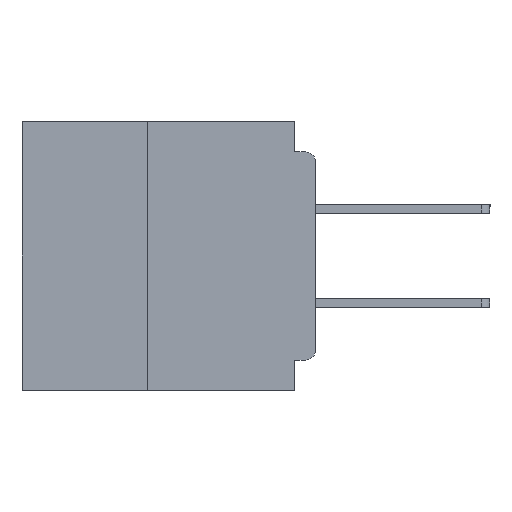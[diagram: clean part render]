
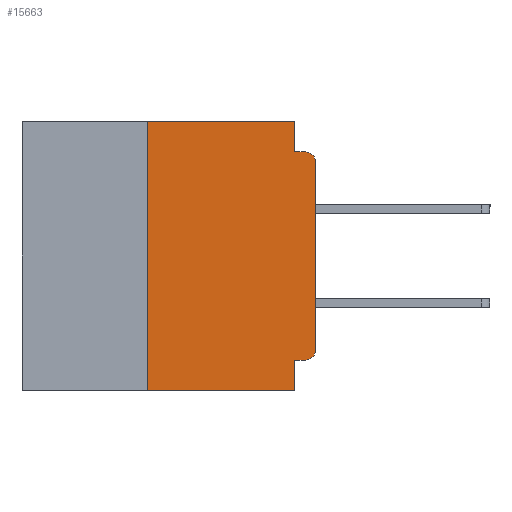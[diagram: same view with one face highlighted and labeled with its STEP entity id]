
A CAD part, left-side view. The second image highlights one B-rep face of the part: STEP entity #15663.
In plain terms, the highlighted planar face has unit normal (-1, 0, 0).
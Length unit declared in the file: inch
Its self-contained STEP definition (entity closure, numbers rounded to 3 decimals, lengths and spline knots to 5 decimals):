
#1507 = FACE_OUTER_BOUND ( 'NONE', #39905, .T. ) ;
#1745 = DIRECTION ( 'NONE',  ( 1., 0., 0. ) ) ;
#2138 = VERTEX_POINT ( 'NONE', #24121 ) ;
#3805 = CIRCLE ( 'NONE', #18743, 0.015 ) ;
#4704 = AXIS2_PLACEMENT_3D ( 'NONE', #35465, #9381, #39820 ) ;
#5245 = VECTOR ( 'NONE', #8273, 39.37008 ) ;
#5449 = VECTOR ( 'NONE', #32065, 39.37008 ) ;
#7479 = LINE ( 'NONE', #47610, #44870 ) ;
#7923 = CARTESIAN_POINT ( 'NONE',  ( 0., 0.031, -0.355 ) ) ;
#8273 = DIRECTION ( 'NONE',  ( 0., -1., 0. ) ) ;
#9055 = VERTEX_POINT ( 'NONE', #28958 ) ;
#9381 = DIRECTION ( 'NONE',  ( -1., 0., 0. ) ) ;
#9544 = VERTEX_POINT ( 'NONE', #45201 ) ;
#9561 = LINE ( 'NONE', #10356, #5449 ) ;
#9749 = ORIENTED_EDGE ( 'NONE', *, *, #20765, .T. ) ;
#10356 = CARTESIAN_POINT ( 'NONE',  ( 0., 0., -0.045 ) ) ;
#10501 = VECTOR ( 'NONE', #42006, 39.37008 ) ;
#11310 = EDGE_CURVE ( 'NONE', #40453, #18278, #43478, .T. ) ;
#11564 = VERTEX_POINT ( 'NONE', #43836 ) ;
#11569 = CARTESIAN_POINT ( 'NONE',  ( 0., 0., 0. ) ) ;
#11880 = LINE ( 'NONE', #11569, #10501 ) ;
#13505 = EDGE_CURVE ( 'NONE', #40234, #40453, #53385, .T. ) ;
#14965 = VERTEX_POINT ( 'NONE', #52963 ) ;
#15224 = ORIENTED_EDGE ( 'NONE', *, *, #13505, .F. ) ;
#15651 = CARTESIAN_POINT ( 'NONE',  ( 0., 0.25, 0. ) ) ;
#15663 = ADVANCED_FACE ( 'NONE', ( #1507 ), #49492, .F. ) ;
#15825 = DIRECTION ( 'NONE',  ( -1., 0., 0. ) ) ;
#16319 = ORIENTED_EDGE ( 'NONE', *, *, #53137, .F. ) ;
#16359 = DIRECTION ( 'NONE',  ( 0., -1., 0. ) ) ;
#17211 = EDGE_CURVE ( 'NONE', #14965, #43392, #7479, .T. ) ;
#18278 = VERTEX_POINT ( 'NONE', #54504 ) ;
#18743 = AXIS2_PLACEMENT_3D ( 'NONE', #41854, #15825, #46175 ) ;
#18803 = VECTOR ( 'NONE', #38897, 39.37008 ) ;
#19768 = EDGE_CURVE ( 'NONE', #14965, #11564, #24973, .T. ) ;
#20765 = EDGE_CURVE ( 'NONE', #11564, #9544, #11880, .T. ) ;
#21612 = VERTEX_POINT ( 'NONE', #34699 ) ;
#21673 = DIRECTION ( 'NONE',  ( 0., 1., 0. ) ) ;
#23966 = EDGE_CURVE ( 'NONE', #43392, #9055, #31575, .T. ) ;
#24121 = CARTESIAN_POINT ( 'NONE',  ( 0., 0.031, -0.045 ) ) ;
#24973 = CIRCLE ( 'NONE', #4704, 0.015 ) ;
#26491 = EDGE_CURVE ( 'NONE', #2138, #21612, #9561, .T. ) ;
#27868 = CARTESIAN_POINT ( 'NONE',  ( 0., 0.437, 0. ) ) ;
#27874 = AXIS2_PLACEMENT_3D ( 'NONE', #27868, #1745, #32235 ) ;
#28591 = ORIENTED_EDGE ( 'NONE', *, *, #17211, .F. ) ;
#28958 = CARTESIAN_POINT ( 'NONE',  ( 0., 0.031, -0.4 ) ) ;
#31353 = CARTESIAN_POINT ( 'NONE',  ( 0., 0.031, -0.4 ) ) ;
#31435 = CARTESIAN_POINT ( 'NONE',  ( 0., 0.25, -0.4 ) ) ;
#31575 = LINE ( 'NONE', #31353, #53280 ) ;
#31953 = ORIENTED_EDGE ( 'NONE', *, *, #49710, .T. ) ;
#32065 = DIRECTION ( 'NONE',  ( 0., -1., 0. ) ) ;
#32087 = VECTOR ( 'NONE', #49600, 39.37008 ) ;
#32235 = DIRECTION ( 'NONE',  ( 0., 0., -1. ) ) ;
#33635 = CARTESIAN_POINT ( 'NONE',  ( 0., 0.437, 0. ) ) ;
#34534 = CARTESIAN_POINT ( 'NONE',  ( 0., 0.25, -0.4 ) ) ;
#34699 = CARTESIAN_POINT ( 'NONE',  ( 0., 0.015, -0.045 ) ) ;
#35465 = CARTESIAN_POINT ( 'NONE',  ( 0., 0.015, -0.34 ) ) ;
#37143 = ORIENTED_EDGE ( 'NONE', *, *, #23966, .F. ) ;
#38897 = DIRECTION ( 'NONE',  ( 0., 0., 1. ) ) ;
#39820 = DIRECTION ( 'NONE',  ( 0., 0., -1. ) ) ;
#39905 = EDGE_LOOP ( 'NONE', ( #9749, #49855, #46845, #16319, #43632, #15224, #31953, #37143, #28591, #56049 ) ) ;
#40096 = DIRECTION ( 'NONE',  ( 0., 0., -1. ) ) ;
#40234 = VERTEX_POINT ( 'NONE', #31435 ) ;
#40453 = VERTEX_POINT ( 'NONE', #15651 ) ;
#41854 = CARTESIAN_POINT ( 'NONE',  ( 0., 0.015, -0.06 ) ) ;
#42006 = DIRECTION ( 'NONE',  ( 0., 0., 1. ) ) ;
#42281 = LINE ( 'NONE', #53946, #32087 ) ;
#43070 = CARTESIAN_POINT ( 'NONE',  ( 0., 0.437, -0.4 ) ) ;
#43392 = VERTEX_POINT ( 'NONE', #7923 ) ;
#43478 = LINE ( 'NONE', #33635, #53651 ) ;
#43632 = ORIENTED_EDGE ( 'NONE', *, *, #11310, .F. ) ;
#43836 = CARTESIAN_POINT ( 'NONE',  ( 0., 0., -0.34 ) ) ;
#44870 = VECTOR ( 'NONE', #21673, 39.37008 ) ;
#45201 = CARTESIAN_POINT ( 'NONE',  ( 0., 0., -0.06 ) ) ;
#46175 = DIRECTION ( 'NONE',  ( 0., 0., -1. ) ) ;
#46845 = ORIENTED_EDGE ( 'NONE', *, *, #26491, .F. ) ;
#47610 = CARTESIAN_POINT ( 'NONE',  ( 0., 0., -0.355 ) ) ;
#49492 = PLANE ( 'NONE',  #27874 ) ;
#49600 = DIRECTION ( 'NONE',  ( 0., 0., -1. ) ) ;
#49710 = EDGE_CURVE ( 'NONE', #40234, #9055, #51511, .T. ) ;
#49855 = ORIENTED_EDGE ( 'NONE', *, *, #55526, .T. ) ;
#51511 = LINE ( 'NONE', #43070, #5245 ) ;
#52963 = CARTESIAN_POINT ( 'NONE',  ( 0., 0.015, -0.355 ) ) ;
#53137 = EDGE_CURVE ( 'NONE', #18278, #2138, #42281, .T. ) ;
#53280 = VECTOR ( 'NONE', #40096, 39.37008 ) ;
#53385 = LINE ( 'NONE', #34534, #18803 ) ;
#53651 = VECTOR ( 'NONE', #16359, 39.37008 ) ;
#53946 = CARTESIAN_POINT ( 'NONE',  ( 0., 0.031, 0. ) ) ;
#54504 = CARTESIAN_POINT ( 'NONE',  ( 0., 0.031, 0. ) ) ;
#55526 = EDGE_CURVE ( 'NONE', #9544, #21612, #3805, .T. ) ;
#56049 = ORIENTED_EDGE ( 'NONE', *, *, #19768, .T. ) ;
